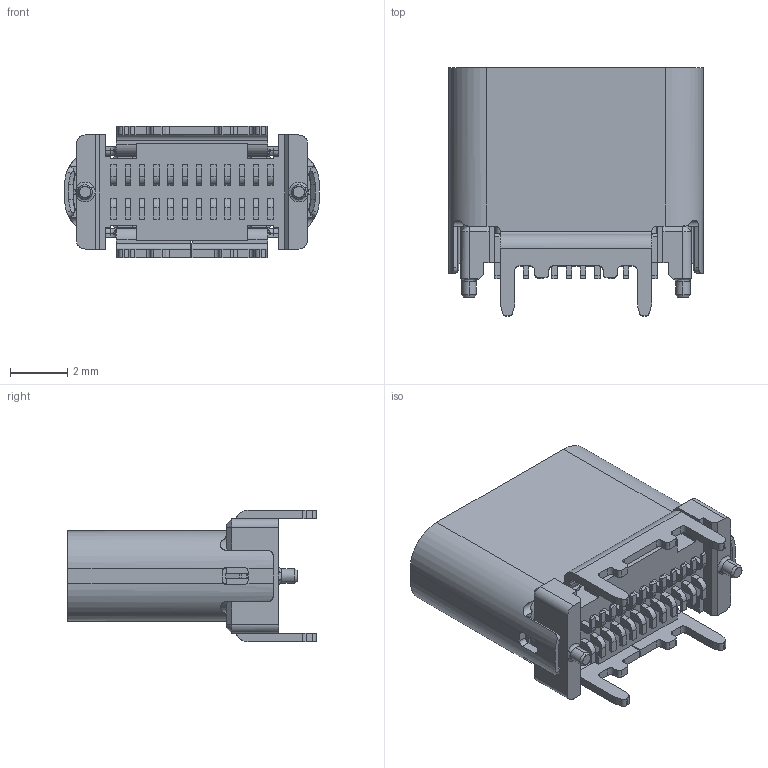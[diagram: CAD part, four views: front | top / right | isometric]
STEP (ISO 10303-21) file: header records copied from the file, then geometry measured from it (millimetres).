
FILE_DESCRIPTION (( 'STEP AP214' ), '1' );
FILE_NAME ('698C124-176-211.STEP', '2021-01-15T17:50:19', ( '' ), ( '' ), 'SwSTEP 2.0', 'SolidWorks 2020', '' );
FILE_SCHEMA (( 'AUTOMOTIVE_DESIGN' ));
Length unit declared in the file: millimetre
Products named in the file (4): Shell2 698C124-176-211; 698C124-176-211; Shell 698C124-176-211; Insulator 698C124-176-211
Assembly tree (3 placements, depth 2):
  698C124-176-211
    Insulator 698C124-176-211
    Shell2 698C124-176-211
    Shell 698C124-176-211
Bounding box: 8.94 x 8.71 x 4.6 mm (x, y, z)
Volume: 122.9 mm3; surface area: 610.9 mm2
Topology: 4 solids, 4 shells, 1222 faces, 3432 edges, 2247 vertices
Faces by surface type: plane 862, cylinder 324, cone 22, bspline 14
Entity records: 45329 total; most frequent: CARTESIAN_POINT 12009, ORIENTED_EDGE 6864, DIRECTION 5168, EDGE_CURVE 3432, VERTEX_POINT 2247, VECTOR 2218, LINE 2218, AXIS2_PLACEMENT_3D 1475
